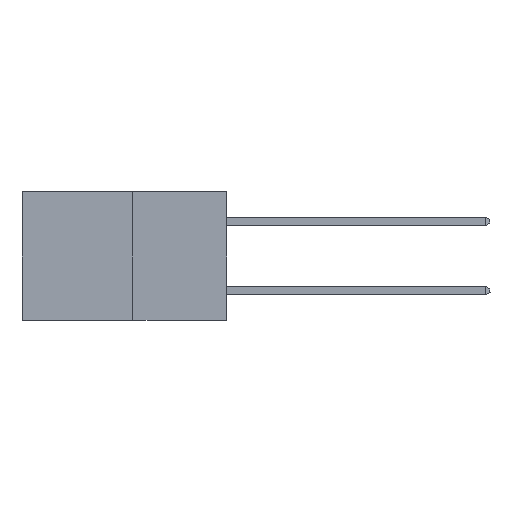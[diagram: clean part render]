
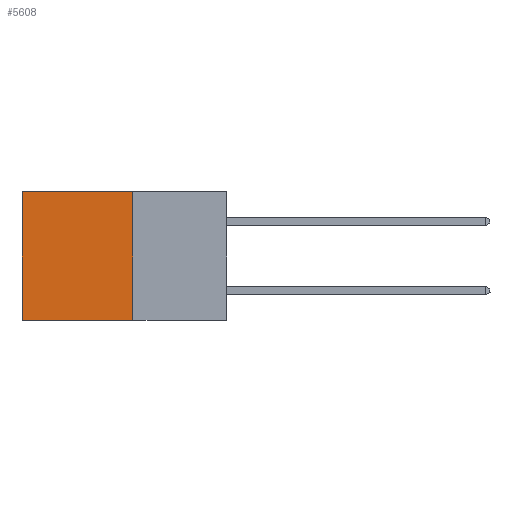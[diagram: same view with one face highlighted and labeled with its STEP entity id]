
A CAD part, left-side view. The second image highlights one B-rep face of the part: STEP entity #5608.
In plain terms, the highlighted planar face has unit normal (-1, 0, 0).
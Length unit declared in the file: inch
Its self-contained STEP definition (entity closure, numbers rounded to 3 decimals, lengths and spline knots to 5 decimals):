
#74 = DIRECTION ( 'NONE',  ( 0., 1., 0. ) ) ;
#462 = DIRECTION ( 'NONE',  ( 0., 0., -1. ) ) ;
#2376 = LINE ( 'NONE', #17793, #6819 ) ;
#2793 = VERTEX_POINT ( 'NONE', #18247 ) ;
#2923 = VECTOR ( 'NONE', #462, 39.37008 ) ;
#4044 = FACE_OUTER_BOUND ( 'NONE', #10000, .T. ) ;
#4047 = CARTESIAN_POINT ( 'NONE',  ( 0.277, 0.27, -0.37 ) ) ;
#4096 = CARTESIAN_POINT ( 'NONE',  ( 0.277, 0.27, 0. ) ) ;
#5608 = ADVANCED_FACE ( 'NONE', ( #4044 ), #6574, .F. ) ;
#6328 = LINE ( 'NONE', #7102, #2923 ) ;
#6574 = PLANE ( 'NONE',  #17715 ) ;
#6819 = VECTOR ( 'NONE', #74, 39.37008 ) ;
#7102 = CARTESIAN_POINT ( 'NONE',  ( 0.277, 0.27, -0.37 ) ) ;
#7575 = DIRECTION ( 'NONE',  ( 1., 0., 0. ) ) ;
#7624 = CARTESIAN_POINT ( 'NONE',  ( 0.277, 0.27, -0.37 ) ) ;
#7723 = VECTOR ( 'NONE', #18422, 39.37008 ) ;
#7808 = DIRECTION ( 'NONE',  ( 0., 0., -1. ) ) ;
#7894 = ORIENTED_EDGE ( 'NONE', *, *, #9585, .F. ) ;
#8789 = ORIENTED_EDGE ( 'NONE', *, *, #9171, .F. ) ;
#9020 = VERTEX_POINT ( 'NONE', #16280 ) ;
#9171 = EDGE_CURVE ( 'NONE', #9020, #12517, #6328, .T. ) ;
#9585 = EDGE_CURVE ( 'NONE', #12517, #12855, #2376, .T. ) ;
#10000 = EDGE_LOOP ( 'NONE', ( #13100, #7894, #8789, #17710 ) ) ;
#11564 = LINE ( 'NONE', #17248, #19827 ) ;
#11938 = DIRECTION ( 'NONE',  ( 0., 0., -1. ) ) ;
#11970 = LINE ( 'NONE', #4096, #7723 ) ;
#12517 = VERTEX_POINT ( 'NONE', #4047 ) ;
#12855 = VERTEX_POINT ( 'NONE', #20679 ) ;
#13100 = ORIENTED_EDGE ( 'NONE', *, *, #15190, .T. ) ;
#15190 = EDGE_CURVE ( 'NONE', #2793, #12855, #11564, .T. ) ;
#16280 = CARTESIAN_POINT ( 'NONE',  ( 0.277, 0.27, 0. ) ) ;
#17248 = CARTESIAN_POINT ( 'NONE',  ( 0.277, 0.59, -0.37 ) ) ;
#17475 = EDGE_CURVE ( 'NONE', #9020, #2793, #11970, .T. ) ;
#17710 = ORIENTED_EDGE ( 'NONE', *, *, #17475, .T. ) ;
#17715 = AXIS2_PLACEMENT_3D ( 'NONE', #7624, #7575, #11938 ) ;
#17793 = CARTESIAN_POINT ( 'NONE',  ( 0.277, 0.27, -0.37 ) ) ;
#18247 = CARTESIAN_POINT ( 'NONE',  ( 0.277, 0.59, 0. ) ) ;
#18422 = DIRECTION ( 'NONE',  ( 0., 1., 0. ) ) ;
#19827 = VECTOR ( 'NONE', #7808, 39.37008 ) ;
#20679 = CARTESIAN_POINT ( 'NONE',  ( 0.277, 0.59, -0.37 ) ) ;
